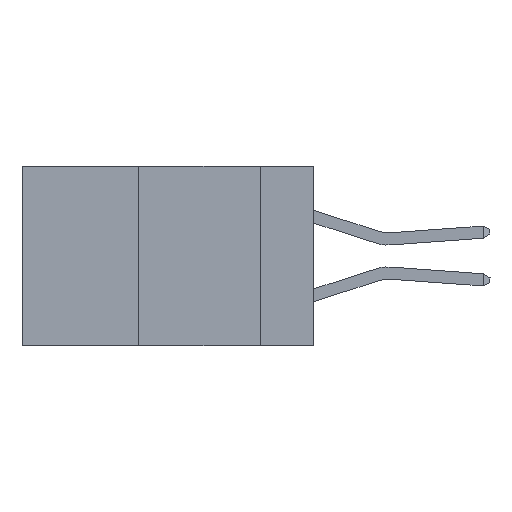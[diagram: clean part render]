
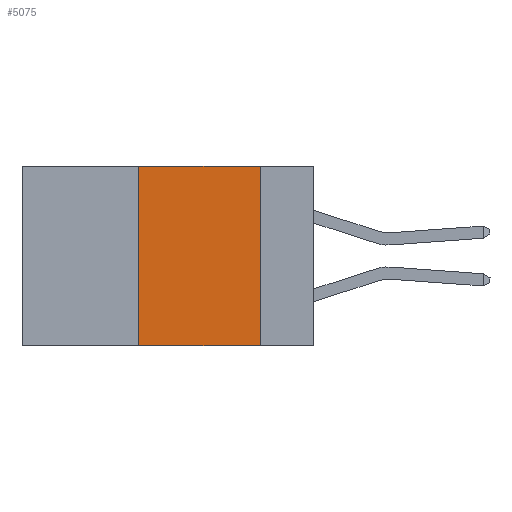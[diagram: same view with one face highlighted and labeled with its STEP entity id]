
A CAD part, left-side view. The second image highlights one B-rep face of the part: STEP entity #5075.
In plain terms, the highlighted planar face has unit normal (-1, 0, 0).
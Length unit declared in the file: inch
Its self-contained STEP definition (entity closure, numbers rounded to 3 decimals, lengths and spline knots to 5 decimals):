
#2213 = DIRECTION ( 'NONE',  ( 0., -1., 0. ) ) ;
#3315 = DIRECTION ( 'NONE',  ( 0., 0., 1. ) ) ;
#5075 = ADVANCED_FACE ( 'NONE', ( #17768 ), #25947, .F. ) ;
#5208 = LINE ( 'NONE', #22305, #21939 ) ;
#6858 = EDGE_CURVE ( 'NONE', #14143, #32997, #5208, .T. ) ;
#7788 = ORIENTED_EDGE ( 'NONE', *, *, #24840, .F. ) ;
#9743 = AXIS2_PLACEMENT_3D ( 'NONE', #14360, #12060, #34667 ) ;
#10361 = DIRECTION ( 'NONE',  ( 0., -1., 0. ) ) ;
#10983 = ORIENTED_EDGE ( 'NONE', *, *, #22402, .F. ) ;
#12058 = LINE ( 'NONE', #26497, #27512 ) ;
#12060 = DIRECTION ( 'NONE',  ( 1., 0., 0. ) ) ;
#14143 = VERTEX_POINT ( 'NONE', #30161 ) ;
#14360 = CARTESIAN_POINT ( 'NONE',  ( 0., 0.6, 0. ) ) ;
#15036 = DIRECTION ( 'NONE',  ( 0., 0., -1. ) ) ;
#16003 = CARTESIAN_POINT ( 'NONE',  ( 0., 0.11, -0.37 ) ) ;
#17703 = CARTESIAN_POINT ( 'NONE',  ( 0., 0.11, 0. ) ) ;
#17768 = FACE_OUTER_BOUND ( 'NONE', #35421, .T. ) ;
#19311 = LINE ( 'NONE', #25392, #29360 ) ;
#21939 = VECTOR ( 'NONE', #10361, 39.37008 ) ;
#22305 = CARTESIAN_POINT ( 'NONE',  ( 0., 0.6, 0. ) ) ;
#22402 = EDGE_CURVE ( 'NONE', #32997, #26765, #34970, .T. ) ;
#24840 = EDGE_CURVE ( 'NONE', #29547, #14143, #12058, .T. ) ;
#25392 = CARTESIAN_POINT ( 'NONE',  ( 0., 0.6, -0.37 ) ) ;
#25726 = CARTESIAN_POINT ( 'NONE',  ( 0., 0.36, -0.37 ) ) ;
#25947 = PLANE ( 'NONE',  #9743 ) ;
#26497 = CARTESIAN_POINT ( 'NONE',  ( 0., 0.36, 0. ) ) ;
#26524 = ORIENTED_EDGE ( 'NONE', *, *, #6858, .F. ) ;
#26765 = VERTEX_POINT ( 'NONE', #16003 ) ;
#27512 = VECTOR ( 'NONE', #3315, 39.37008 ) ;
#27849 = EDGE_CURVE ( 'NONE', #29547, #26765, #19311, .T. ) ;
#29360 = VECTOR ( 'NONE', #2213, 39.37008 ) ;
#29547 = VERTEX_POINT ( 'NONE', #25726 ) ;
#30161 = CARTESIAN_POINT ( 'NONE',  ( 0., 0.36, 0. ) ) ;
#31298 = ORIENTED_EDGE ( 'NONE', *, *, #27849, .T. ) ;
#32997 = VERTEX_POINT ( 'NONE', #17703 ) ;
#34031 = VECTOR ( 'NONE', #15036, 39.37008 ) ;
#34667 = DIRECTION ( 'NONE',  ( 0., 0., -1. ) ) ;
#34970 = LINE ( 'NONE', #35149, #34031 ) ;
#35149 = CARTESIAN_POINT ( 'NONE',  ( 0., 0.11, 0. ) ) ;
#35421 = EDGE_LOOP ( 'NONE', ( #10983, #26524, #7788, #31298 ) ) ;
